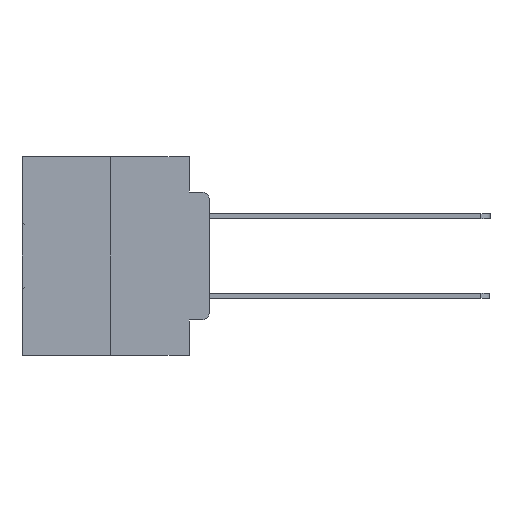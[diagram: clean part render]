
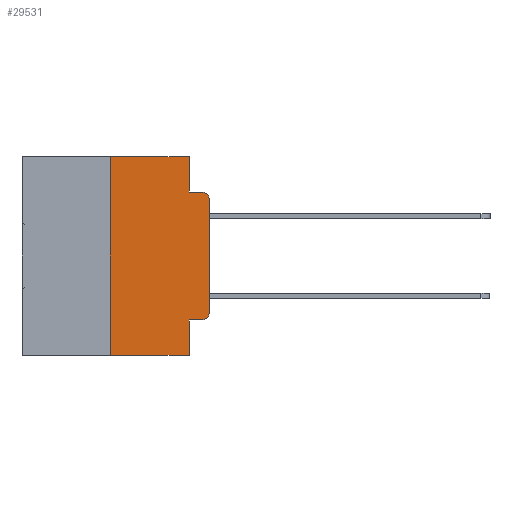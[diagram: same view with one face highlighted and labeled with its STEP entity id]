
A CAD part, left-side view. The second image highlights one B-rep face of the part: STEP entity #29531.
In plain terms, the highlighted planar face has unit normal (-1, 0, 0).
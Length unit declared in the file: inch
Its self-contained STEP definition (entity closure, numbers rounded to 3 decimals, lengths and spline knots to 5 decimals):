
#193 = CARTESIAN_POINT ( 'NONE',  ( 0., 0.02, -0.0885 ) ) ;
#1058 = EDGE_CURVE ( 'NONE', #22541, #18629, #17820, .T. ) ;
#2460 = PLANE ( 'NONE',  #23643 ) ;
#2563 = ORIENTED_EDGE ( 'NONE', *, *, #20122, .F. ) ;
#3425 = LINE ( 'NONE', #26047, #16193 ) ;
#3989 = LINE ( 'NONE', #32540, #29993 ) ;
#4220 = CARTESIAN_POINT ( 'NONE',  ( 0., 0., -0.1085 ) ) ;
#4841 = LINE ( 'NONE', #14714, #10777 ) ;
#5019 = VECTOR ( 'NONE', #25980, 39.37008 ) ;
#5420 = DIRECTION ( 'NONE',  ( 0., 0., -1. ) ) ;
#5864 = DIRECTION ( 'NONE',  ( 0., 0., -1. ) ) ;
#5910 = CARTESIAN_POINT ( 'NONE',  ( 0., 0.25, 0. ) ) ;
#6231 = ORIENTED_EDGE ( 'NONE', *, *, #1058, .T. ) ;
#6391 = AXIS2_PLACEMENT_3D ( 'NONE', #10865, #28443, #13465 ) ;
#6750 = EDGE_CURVE ( 'NONE', #10403, #32697, #11788, .T. ) ;
#7122 = DIRECTION ( 'NONE',  ( 0., -1., 0. ) ) ;
#8169 = LINE ( 'NONE', #5910, #13348 ) ;
#8577 = ORIENTED_EDGE ( 'NONE', *, *, #15473, .T. ) ;
#9061 = VERTEX_POINT ( 'NONE', #24094 ) ;
#9533 = VERTEX_POINT ( 'NONE', #16016 ) ;
#10403 = VERTEX_POINT ( 'NONE', #24448 ) ;
#10544 = ORIENTED_EDGE ( 'NONE', *, *, #22198, .F. ) ;
#10777 = VECTOR ( 'NONE', #7122, 39.37008 ) ;
#10865 = CARTESIAN_POINT ( 'NONE',  ( 0., 0.02, -0.3915 ) ) ;
#11123 = DIRECTION ( 'NONE',  ( -1., 0., 0. ) ) ;
#11450 = CARTESIAN_POINT ( 'NONE',  ( 0., 0.25, 0. ) ) ;
#11788 = LINE ( 'NONE', #13069, #5019 ) ;
#12347 = EDGE_LOOP ( 'NONE', ( #6231, #13012, #14629, #22064, #2563, #15726, #23188, #10544, #17564, #8577 ) ) ;
#12743 = VERTEX_POINT ( 'NONE', #11450 ) ;
#13012 = ORIENTED_EDGE ( 'NONE', *, *, #32127, .T. ) ;
#13069 = CARTESIAN_POINT ( 'NONE',  ( 0., 0.473, -0.5 ) ) ;
#13225 = CARTESIAN_POINT ( 'NONE',  ( 0., 0.051, -0.5 ) ) ;
#13348 = VECTOR ( 'NONE', #18530, 39.37008 ) ;
#13465 = DIRECTION ( 'NONE',  ( 0., 0., -1. ) ) ;
#13497 = CARTESIAN_POINT ( 'NONE',  ( 0., 0.051, -0.4115 ) ) ;
#13570 = LINE ( 'NONE', #26113, #26101 ) ;
#13629 = DIRECTION ( 'NONE',  ( 0., 0., -1. ) ) ;
#14629 = ORIENTED_EDGE ( 'NONE', *, *, #28850, .F. ) ;
#14692 = DIRECTION ( 'NONE',  ( 0., 0., 1. ) ) ;
#14714 = CARTESIAN_POINT ( 'NONE',  ( 0., 0.051, -0.4115 ) ) ;
#15260 = CARTESIAN_POINT ( 'NONE',  ( 0., 0.473, 0. ) ) ;
#15473 = EDGE_CURVE ( 'NONE', #9061, #22541, #25501, .T. ) ;
#15726 = ORIENTED_EDGE ( 'NONE', *, *, #23903, .F. ) ;
#16016 = CARTESIAN_POINT ( 'NONE',  ( 0., 0.051, -0.0885 ) ) ;
#16193 = VECTOR ( 'NONE', #5864, 39.37008 ) ;
#16306 = AXIS2_PLACEMENT_3D ( 'NONE', #26217, #11123, #28692 ) ;
#17034 = VECTOR ( 'NONE', #14692, 39.37008 ) ;
#17122 = EDGE_CURVE ( 'NONE', #23911, #9061, #4841, .T. ) ;
#17400 = CARTESIAN_POINT ( 'NONE',  ( 0., 0.051, 0. ) ) ;
#17564 = ORIENTED_EDGE ( 'NONE', *, *, #17122, .T. ) ;
#17820 = LINE ( 'NONE', #19515, #17034 ) ;
#18530 = DIRECTION ( 'NONE',  ( 0., 0., 1. ) ) ;
#18629 = VERTEX_POINT ( 'NONE', #4220 ) ;
#19515 = CARTESIAN_POINT ( 'NONE',  ( 0., 0., 0. ) ) ;
#19997 = CARTESIAN_POINT ( 'NONE',  ( 0., 0.051, -0.0885 ) ) ;
#20122 = EDGE_CURVE ( 'NONE', #12743, #24298, #3989, .T. ) ;
#20564 = DIRECTION ( 'NONE',  ( 1., 0., 0. ) ) ;
#20708 = VERTEX_POINT ( 'NONE', #193 ) ;
#22064 = ORIENTED_EDGE ( 'NONE', *, *, #27208, .F. ) ;
#22198 = EDGE_CURVE ( 'NONE', #23911, #32697, #3425, .T. ) ;
#22541 = VERTEX_POINT ( 'NONE', #29802 ) ;
#22726 = DIRECTION ( 'NONE',  ( 0., -1., 0. ) ) ;
#23188 = ORIENTED_EDGE ( 'NONE', *, *, #6750, .T. ) ;
#23643 = AXIS2_PLACEMENT_3D ( 'NONE', #15260, #20564, #5420 ) ;
#23903 = EDGE_CURVE ( 'NONE', #10403, #12743, #8169, .T. ) ;
#23911 = VERTEX_POINT ( 'NONE', #13497 ) ;
#24094 = CARTESIAN_POINT ( 'NONE',  ( 0., 0.02, -0.4115 ) ) ;
#24298 = VERTEX_POINT ( 'NONE', #17400 ) ;
#24448 = CARTESIAN_POINT ( 'NONE',  ( 0., 0.25, -0.5 ) ) ;
#25501 = CIRCLE ( 'NONE', #6391, 0.02 ) ;
#25610 = LINE ( 'NONE', #19997, #31347 ) ;
#25980 = DIRECTION ( 'NONE',  ( 0., -1., 0. ) ) ;
#26047 = CARTESIAN_POINT ( 'NONE',  ( 0., 0.051, 0. ) ) ;
#26101 = VECTOR ( 'NONE', #13629, 39.37008 ) ;
#26113 = CARTESIAN_POINT ( 'NONE',  ( 0., 0.051, 0. ) ) ;
#26217 = CARTESIAN_POINT ( 'NONE',  ( 0., 0.02, -0.1085 ) ) ;
#27208 = EDGE_CURVE ( 'NONE', #24298, #9533, #13570, .T. ) ;
#27271 = CIRCLE ( 'NONE', #16306, 0.02 ) ;
#27522 = DIRECTION ( 'NONE',  ( 0., -1., 0. ) ) ;
#28443 = DIRECTION ( 'NONE',  ( -1., 0., 0. ) ) ;
#28692 = DIRECTION ( 'NONE',  ( 0., 0., -1. ) ) ;
#28850 = EDGE_CURVE ( 'NONE', #9533, #20708, #25610, .T. ) ;
#29531 = ADVANCED_FACE ( 'NONE', ( #32473 ), #2460, .F. ) ;
#29802 = CARTESIAN_POINT ( 'NONE',  ( 0., 0., -0.3915 ) ) ;
#29993 = VECTOR ( 'NONE', #22726, 39.37008 ) ;
#31347 = VECTOR ( 'NONE', #27522, 39.37008 ) ;
#32127 = EDGE_CURVE ( 'NONE', #18629, #20708, #27271, .T. ) ;
#32473 = FACE_OUTER_BOUND ( 'NONE', #12347, .T. ) ;
#32540 = CARTESIAN_POINT ( 'NONE',  ( 0., 0.473, 0. ) ) ;
#32697 = VERTEX_POINT ( 'NONE', #13225 ) ;
